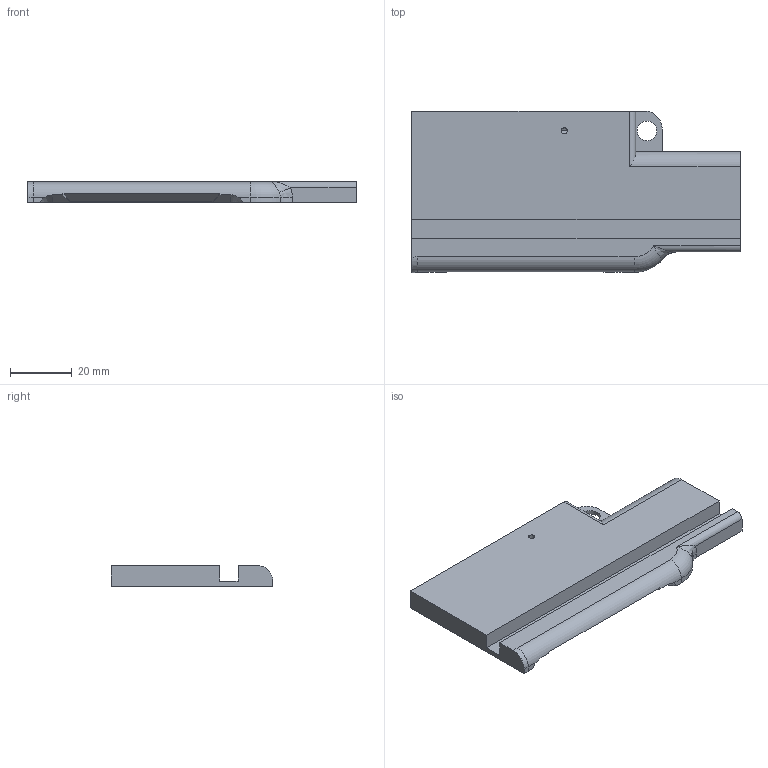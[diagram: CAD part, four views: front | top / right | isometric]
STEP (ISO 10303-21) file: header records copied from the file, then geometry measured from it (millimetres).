
FILE_DESCRIPTION (( 'STEP AP214' ), '1' );
FILE_NAME ('Receiver_Magwell_Right.step', '2014-05-14T06:10:18', ( 'WarFairy' ), ( '' ), 'SwSTEP 2.0', 'SolidWorks 2013', '' );
FILE_SCHEMA (( 'AUTOMOTIVE_DESIGN' ));
Length unit declared in the file: inch
Products named in the file (1): Receiver_Magwell_Right
Bounding box: 106.45 x 52.34 x 6.72 mm (x, y, z)
Volume: 28841.5 mm3; surface area: 12960.1 mm2
Topology: 1 solids, 1 shells, 46 faces, 127 edges, 80 vertices
Faces by surface type: plane 21, cylinder 17, cone 4, torus 2, bspline 2
Entity records: 1696 total; most frequent: CARTESIAN_POINT 512, ORIENTED_EDGE 248, DIRECTION 227, EDGE_CURVE 124, VERTEX_POINT 80, AXIS2_PLACEMENT_3D 76, VECTOR 75, LINE 75
